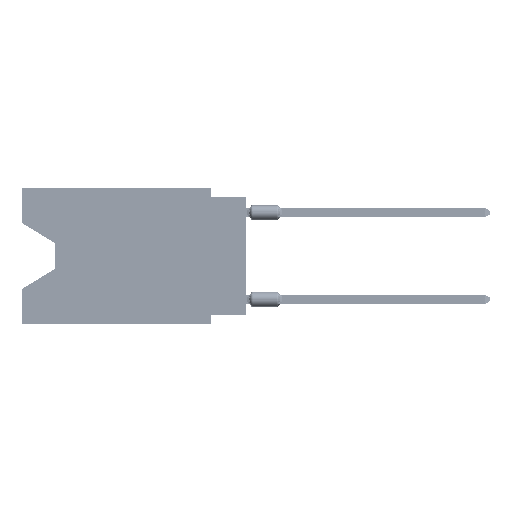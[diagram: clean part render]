
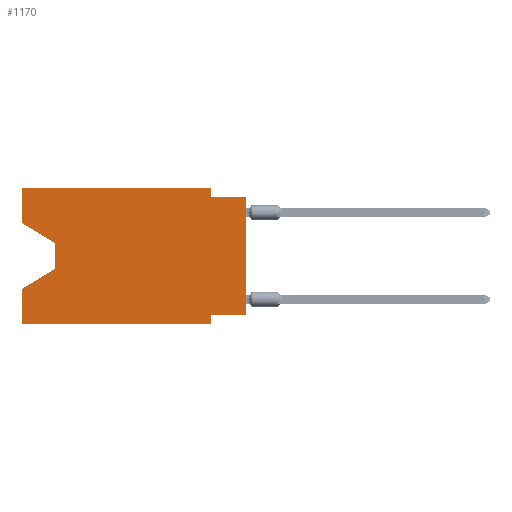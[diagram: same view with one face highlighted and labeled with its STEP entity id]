
A CAD part, left-side view. The second image highlights one B-rep face of the part: STEP entity #1170.
In plain terms, the highlighted planar face has unit normal (-1, 0, 0).
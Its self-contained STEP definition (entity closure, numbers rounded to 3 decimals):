
#632 = AXIS2_PLACEMENT_3D ( 'NONE', #50280, #67286, #32571 ) ;
#1170 = ADVANCED_FACE ( 'NONE', ( #27631 ), #15917, .F. ) ;
#1234 = DIRECTION ( 'NONE',  ( 0., -1., 0. ) ) ;
#1594 = ORIENTED_EDGE ( 'NONE', *, *, #46758, .F. ) ;
#1677 = VERTEX_POINT ( 'NONE', #33588 ) ;
#2622 = EDGE_CURVE ( 'NONE', #68897, #54771, #36673, .T. ) ;
#3472 = DIRECTION ( 'NONE',  ( 0., 0., -1. ) ) ;
#3653 = CARTESIAN_POINT ( 'NONE',  ( 0., 13.97, -5.893 ) ) ;
#3762 = VECTOR ( 'NONE', #48097, 1000. ) ;
#3947 = CARTESIAN_POINT ( 'NONE',  ( 0., 13.97, -4.013 ) ) ;
#4554 = CARTESIAN_POINT ( 'NONE',  ( 0., 2.54, 0. ) ) ;
#4833 = CARTESIAN_POINT ( 'NONE',  ( 0., 16.383, -9.906 ) ) ;
#6047 = DIRECTION ( 'NONE',  ( 0., 0., -1. ) ) ;
#6504 = VECTOR ( 'NONE', #57341, 1000. ) ;
#7404 = DIRECTION ( 'NONE',  ( 0., -1., 0. ) ) ;
#8636 = LINE ( 'NONE', #66783, #61563 ) ;
#9186 = VERTEX_POINT ( 'NONE', #3653 ) ;
#11428 = VECTOR ( 'NONE', #53273, 1000. ) ;
#11447 = LINE ( 'NONE', #69215, #74407 ) ;
#12036 = CARTESIAN_POINT ( 'NONE',  ( 0., 16.383, 0. ) ) ;
#12491 = CARTESIAN_POINT ( 'NONE',  ( 0., 16.383, 0. ) ) ;
#13738 = LINE ( 'NONE', #48465, #3762 ) ;
#14145 = EDGE_CURVE ( 'NONE', #60365, #41961, #54448, .T. ) ;
#14175 = VERTEX_POINT ( 'NONE', #26511 ) ;
#15542 = VERTEX_POINT ( 'NONE', #34053 ) ;
#15752 = VERTEX_POINT ( 'NONE', #64970 ) ;
#15917 = PLANE ( 'NONE',  #632 ) ;
#16792 = CARTESIAN_POINT ( 'NONE',  ( 0., 2.54, -9.906 ) ) ;
#16814 = ORIENTED_EDGE ( 'NONE', *, *, #21948, .T. ) ;
#16869 = CARTESIAN_POINT ( 'NONE',  ( 0., 2.54, -9.271 ) ) ;
#19620 = VECTOR ( 'NONE', #6047, 1000. ) ;
#20100 = EDGE_CURVE ( 'NONE', #61392, #1677, #57770, .T. ) ;
#20213 = DIRECTION ( 'NONE',  ( 0., 0., -1. ) ) ;
#20352 = DIRECTION ( 'NONE',  ( 0., 0., 1. ) ) ;
#21948 = EDGE_CURVE ( 'NONE', #9186, #54771, #47501, .T. ) ;
#22639 = LINE ( 'NONE', #12036, #39730 ) ;
#24209 = DIRECTION ( 'NONE',  ( 0., 0., 1. ) ) ;
#25806 = VECTOR ( 'NONE', #36307, 1000. ) ;
#26511 = CARTESIAN_POINT ( 'NONE',  ( 0., 0., -9.271 ) ) ;
#26652 = ORIENTED_EDGE ( 'NONE', *, *, #43330, .F. ) ;
#27631 = FACE_OUTER_BOUND ( 'NONE', #51804, .T. ) ;
#27858 = EDGE_CURVE ( 'NONE', #56500, #15542, #58177, .T. ) ;
#32196 = VECTOR ( 'NONE', #24209, 1000. ) ;
#32571 = DIRECTION ( 'NONE',  ( 0., 0., -1. ) ) ;
#32903 = EDGE_CURVE ( 'NONE', #15542, #9186, #48888, .T. ) ;
#33588 = CARTESIAN_POINT ( 'NONE',  ( 0., 2.54, -0.635 ) ) ;
#34053 = CARTESIAN_POINT ( 'NONE',  ( 0., 13.97, -4.013 ) ) ;
#36307 = DIRECTION ( 'NONE',  ( 0., 0., 1. ) ) ;
#36673 = LINE ( 'NONE', #41566, #32196 ) ;
#36879 = CARTESIAN_POINT ( 'NONE',  ( 0., 0., -0.635 ) ) ;
#37020 = ORIENTED_EDGE ( 'NONE', *, *, #41238, .F. ) ;
#37850 = CARTESIAN_POINT ( 'NONE',  ( 0., 2.54, -9.906 ) ) ;
#39583 = VECTOR ( 'NONE', #20213, 1000. ) ;
#39730 = VECTOR ( 'NONE', #45650, 1000. ) ;
#40141 = VERTEX_POINT ( 'NONE', #73629 ) ;
#41238 = EDGE_CURVE ( 'NONE', #15752, #61392, #22639, .T. ) ;
#41566 = CARTESIAN_POINT ( 'NONE',  ( 0., 16.383, 0. ) ) ;
#41671 = CARTESIAN_POINT ( 'NONE',  ( 0., 16.383, -7.36 ) ) ;
#41961 = VERTEX_POINT ( 'NONE', #16792 ) ;
#42516 = LINE ( 'NONE', #36879, #63169 ) ;
#43330 = EDGE_CURVE ( 'NONE', #14175, #60365, #13738, .T. ) ;
#45650 = DIRECTION ( 'NONE',  ( 0., -1., 0. ) ) ;
#45687 = ORIENTED_EDGE ( 'NONE', *, *, #55618, .F. ) ;
#46374 = CARTESIAN_POINT ( 'NONE',  ( 0., 13.97, -5.893 ) ) ;
#46758 = EDGE_CURVE ( 'NONE', #56500, #15752, #47599, .T. ) ;
#47501 = LINE ( 'NONE', #46374, #6504 ) ;
#47599 = LINE ( 'NONE', #12491, #25806 ) ;
#48097 = DIRECTION ( 'NONE',  ( 0., 1., 0. ) ) ;
#48351 = CARTESIAN_POINT ( 'NONE',  ( 0., 2.54, 0. ) ) ;
#48465 = CARTESIAN_POINT ( 'NONE',  ( 0., 0., -9.271 ) ) ;
#48753 = ORIENTED_EDGE ( 'NONE', *, *, #32903, .T. ) ;
#48888 = LINE ( 'NONE', #3947, #39583 ) ;
#49879 = CARTESIAN_POINT ( 'NONE',  ( 0., 16.383, -2.546 ) ) ;
#50280 = CARTESIAN_POINT ( 'NONE',  ( 0., 16.383, 0. ) ) ;
#51627 = ORIENTED_EDGE ( 'NONE', *, *, #27858, .T. ) ;
#51797 = ORIENTED_EDGE ( 'NONE', *, *, #73019, .T. ) ;
#51804 = EDGE_LOOP ( 'NONE', ( #51627, #48753, #16814, #72178, #51797, #64542, #26652, #55840, #45687, #71680, #37020, #1594 ) ) ;
#51902 = EDGE_CURVE ( 'NONE', #14175, #40141, #8636, .T. ) ;
#53273 = DIRECTION ( 'NONE',  ( 0., -0.855, -0.519 ) ) ;
#54448 = LINE ( 'NONE', #37850, #58837 ) ;
#54771 = VERTEX_POINT ( 'NONE', #41671 ) ;
#55618 = EDGE_CURVE ( 'NONE', #1677, #40141, #42516, .T. ) ;
#55840 = ORIENTED_EDGE ( 'NONE', *, *, #51902, .T. ) ;
#56500 = VERTEX_POINT ( 'NONE', #49879 ) ;
#57341 = DIRECTION ( 'NONE',  ( 0., 0.855, -0.519 ) ) ;
#57770 = LINE ( 'NONE', #4554, #19620 ) ;
#58177 = LINE ( 'NONE', #74167, #11428 ) ;
#58837 = VECTOR ( 'NONE', #3472, 1000. ) ;
#60365 = VERTEX_POINT ( 'NONE', #16869 ) ;
#61392 = VERTEX_POINT ( 'NONE', #48351 ) ;
#61563 = VECTOR ( 'NONE', #20352, 1000. ) ;
#63169 = VECTOR ( 'NONE', #7404, 1000. ) ;
#64542 = ORIENTED_EDGE ( 'NONE', *, *, #14145, .F. ) ;
#64970 = CARTESIAN_POINT ( 'NONE',  ( 0., 16.383, 0. ) ) ;
#66783 = CARTESIAN_POINT ( 'NONE',  ( 0., 0., 0. ) ) ;
#67286 = DIRECTION ( 'NONE',  ( 1., 0., 0. ) ) ;
#68897 = VERTEX_POINT ( 'NONE', #4833 ) ;
#69215 = CARTESIAN_POINT ( 'NONE',  ( 0., 16.383, -9.906 ) ) ;
#71680 = ORIENTED_EDGE ( 'NONE', *, *, #20100, .F. ) ;
#72178 = ORIENTED_EDGE ( 'NONE', *, *, #2622, .F. ) ;
#73019 = EDGE_CURVE ( 'NONE', #68897, #41961, #11447, .T. ) ;
#73629 = CARTESIAN_POINT ( 'NONE',  ( 0., 0., -0.635 ) ) ;
#74167 = CARTESIAN_POINT ( 'NONE',  ( 0., 16.383, -2.546 ) ) ;
#74407 = VECTOR ( 'NONE', #1234, 1000. ) ;
